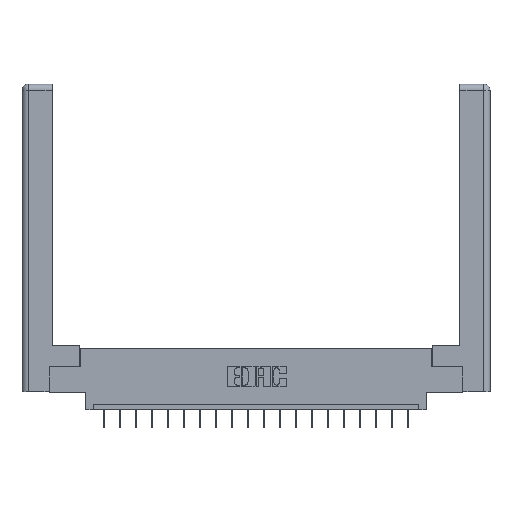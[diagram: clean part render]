
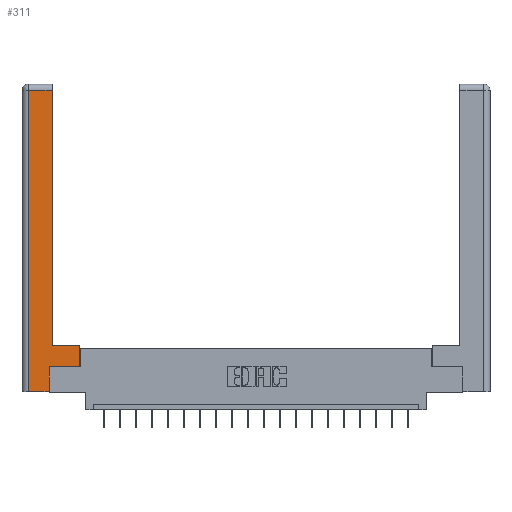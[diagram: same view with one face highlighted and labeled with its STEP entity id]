
A CAD part, top view. The second image highlights one B-rep face of the part: STEP entity #311.
In plain terms, the highlighted planar face has unit normal (0, 0, 1).
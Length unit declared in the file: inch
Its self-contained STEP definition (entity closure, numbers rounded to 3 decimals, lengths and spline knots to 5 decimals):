
#51 = VERTEX_POINT ( 'NONE', #1105 ) ;
#311 = ADVANCED_FACE ( 'NONE', ( #16319 ), #4145, .F. ) ;
#1087 = CARTESIAN_POINT ( 'NONE',  ( 0.565, 0.245, 0. ) ) ;
#1105 = CARTESIAN_POINT ( 'NONE',  ( 0.565, 0.45, 0. ) ) ;
#1154 = EDGE_CURVE ( 'NONE', #3918, #18805, #1419, .T. ) ;
#1419 = LINE ( 'NONE', #20373, #2677 ) ;
#1570 = ORIENTED_EDGE ( 'NONE', *, *, #10738, .T. ) ;
#1652 = LINE ( 'NONE', #1087, #11083 ) ;
#1657 = EDGE_CURVE ( 'NONE', #20027, #4633, #1652, .T. ) ;
#1835 = ORIENTED_EDGE ( 'NONE', *, *, #12371, .T. ) ;
#2149 = VECTOR ( 'NONE', #14201, 39.37008 ) ;
#2274 = CARTESIAN_POINT ( 'NONE',  ( 0.295, 2.94, 0. ) ) ;
#2677 = VECTOR ( 'NONE', #15471, 39.37008 ) ;
#2849 = VERTEX_POINT ( 'NONE', #7142 ) ;
#3357 = CARTESIAN_POINT ( 'NONE',  ( 0.265, 0.245, 0. ) ) ;
#3918 = VERTEX_POINT ( 'NONE', #13928 ) ;
#4145 = PLANE ( 'NONE',  #16711 ) ;
#4170 = DIRECTION ( 'NONE',  ( 0., 1., 0. ) ) ;
#4633 = VERTEX_POINT ( 'NONE', #9247 ) ;
#5593 = CARTESIAN_POINT ( 'NONE',  ( 0.0615, 0., 0. ) ) ;
#5599 = VECTOR ( 'NONE', #4170, 39.37008 ) ;
#5720 = ORIENTED_EDGE ( 'NONE', *, *, #1154, .T. ) ;
#5744 = DIRECTION ( 'NONE',  ( 1., 0., 0. ) ) ;
#6198 = CARTESIAN_POINT ( 'NONE',  ( 0.265, 0.245, 0. ) ) ;
#6463 = DIRECTION ( 'NONE',  ( -1., 0., 0. ) ) ;
#6465 = VERTEX_POINT ( 'NONE', #2274 ) ;
#6883 = CARTESIAN_POINT ( 'NONE',  ( 0.295, 0.45, 0. ) ) ;
#7142 = CARTESIAN_POINT ( 'NONE',  ( 0.265, 0., 0. ) ) ;
#7412 = DIRECTION ( 'NONE',  ( 0., 0., -1. ) ) ;
#7570 = LINE ( 'NONE', #14636, #5599 ) ;
#7915 = ORIENTED_EDGE ( 'NONE', *, *, #13034, .T. ) ;
#8065 = LINE ( 'NONE', #20514, #9554 ) ;
#9045 = CARTESIAN_POINT ( 'NONE',  ( 0.265, 0., 0. ) ) ;
#9142 = VERTEX_POINT ( 'NONE', #6883 ) ;
#9247 = CARTESIAN_POINT ( 'NONE',  ( 0.565, 0.245, 0. ) ) ;
#9352 = EDGE_CURVE ( 'NONE', #4633, #51, #7570, .T. ) ;
#9554 = VECTOR ( 'NONE', #15811, 39.37008 ) ;
#9817 = VECTOR ( 'NONE', #6463, 39.37008 ) ;
#10005 = CARTESIAN_POINT ( 'NONE',  ( 0.295, 3., 0. ) ) ;
#10738 = EDGE_CURVE ( 'NONE', #9142, #6465, #19262, .T. ) ;
#11083 = VECTOR ( 'NONE', #20018, 39.37008 ) ;
#11468 = DIRECTION ( 'NONE',  ( 0., 1., 0. ) ) ;
#11486 = ORIENTED_EDGE ( 'NONE', *, *, #9352, .T. ) ;
#11551 = ORIENTED_EDGE ( 'NONE', *, *, #16096, .T. ) ;
#12371 = EDGE_CURVE ( 'NONE', #2849, #20027, #19254, .T. ) ;
#12932 = EDGE_CURVE ( 'NONE', #6465, #3918, #19236, .T. ) ;
#13034 = EDGE_CURVE ( 'NONE', #51, #9142, #8065, .T. ) ;
#13150 = LINE ( 'NONE', #9045, #20081 ) ;
#13461 = ORIENTED_EDGE ( 'NONE', *, *, #12932, .T. ) ;
#13928 = CARTESIAN_POINT ( 'NONE',  ( 0.0615, 2.94, 0. ) ) ;
#14201 = DIRECTION ( 'NONE',  ( 0., 1., 0. ) ) ;
#14636 = CARTESIAN_POINT ( 'NONE',  ( 0.565, 0.45, 0. ) ) ;
#14923 = ORIENTED_EDGE ( 'NONE', *, *, #1657, .T. ) ;
#15023 = CARTESIAN_POINT ( 'NONE',  ( 0.0615, 2.94, 0. ) ) ;
#15471 = DIRECTION ( 'NONE',  ( 0., -1., 0. ) ) ;
#15811 = DIRECTION ( 'NONE',  ( -1., 0., 0. ) ) ;
#16096 = EDGE_CURVE ( 'NONE', #18805, #2849, #13150, .T. ) ;
#16319 = FACE_OUTER_BOUND ( 'NONE', #19084, .T. ) ;
#16711 = AXIS2_PLACEMENT_3D ( 'NONE', #20068, #7412, #16817 ) ;
#16817 = DIRECTION ( 'NONE',  ( -1., 0., 0. ) ) ;
#18277 = VECTOR ( 'NONE', #11468, 39.37008 ) ;
#18805 = VERTEX_POINT ( 'NONE', #5593 ) ;
#19084 = EDGE_LOOP ( 'NONE', ( #1570, #13461, #5720, #11551, #1835, #14923, #11486, #7915 ) ) ;
#19236 = LINE ( 'NONE', #15023, #9817 ) ;
#19254 = LINE ( 'NONE', #6198, #2149 ) ;
#19262 = LINE ( 'NONE', #10005, #18277 ) ;
#20018 = DIRECTION ( 'NONE',  ( 1., 0., 0. ) ) ;
#20027 = VERTEX_POINT ( 'NONE', #3357 ) ;
#20068 = CARTESIAN_POINT ( 'NONE',  ( 0., 0., 0. ) ) ;
#20081 = VECTOR ( 'NONE', #5744, 39.37008 ) ;
#20373 = CARTESIAN_POINT ( 'NONE',  ( 0.0615, 0., 0. ) ) ;
#20514 = CARTESIAN_POINT ( 'NONE',  ( 0.295, 0.45, 0. ) ) ;
